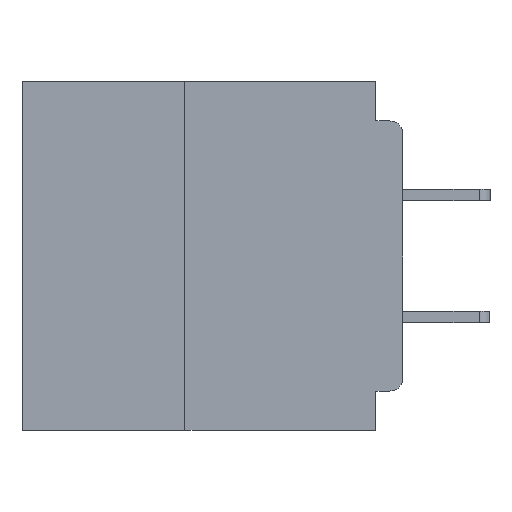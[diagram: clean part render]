
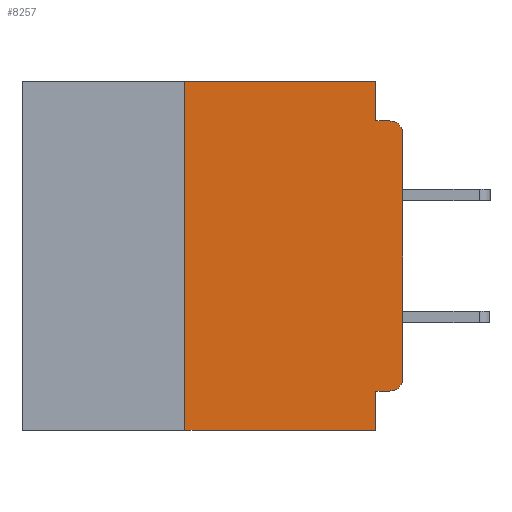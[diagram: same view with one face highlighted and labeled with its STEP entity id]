
A CAD part, left-side view. The second image highlights one B-rep face of the part: STEP entity #8257.
In plain terms, the highlighted planar face has unit normal (-1, 0, 0).
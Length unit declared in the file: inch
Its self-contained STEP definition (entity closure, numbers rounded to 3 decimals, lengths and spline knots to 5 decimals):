
#768 = EDGE_CURVE ( 'NONE', #29755, #1207, #26819, .T. ) ;
#1207 = VERTEX_POINT ( 'NONE', #32233 ) ;
#1720 = VERTEX_POINT ( 'NONE', #8453 ) ;
#1744 = CARTESIAN_POINT ( 'NONE',  ( 0., 0.031, -0.355 ) ) ;
#4543 = EDGE_CURVE ( 'NONE', #17490, #6788, #8308, .T. ) ;
#4868 = CARTESIAN_POINT ( 'NONE',  ( 0., 0., -0.34 ) ) ;
#5256 = ORIENTED_EDGE ( 'NONE', *, *, #768, .F. ) ;
#5502 = CIRCLE ( 'NONE', #35044, 0.015 ) ;
#6087 = LINE ( 'NONE', #44085, #14259 ) ;
#6788 = VERTEX_POINT ( 'NONE', #32227 ) ;
#6913 = ORIENTED_EDGE ( 'NONE', *, *, #19976, .F. ) ;
#7163 = DIRECTION ( 'NONE',  ( 0., 1., 0. ) ) ;
#7928 = VERTEX_POINT ( 'NONE', #41625 ) ;
#8257 = ADVANCED_FACE ( 'NONE', ( #42721 ), #23032, .F. ) ;
#8308 = LINE ( 'NONE', #13569, #34589 ) ;
#8453 = CARTESIAN_POINT ( 'NONE',  ( 0., 0.015, -0.355 ) ) ;
#9027 = VERTEX_POINT ( 'NONE', #23716 ) ;
#9641 = ORIENTED_EDGE ( 'NONE', *, *, #42508, .F. ) ;
#10364 = CARTESIAN_POINT ( 'NONE',  ( 0., 0.031, 0. ) ) ;
#10952 = EDGE_CURVE ( 'NONE', #1720, #43732, #23913, .T. ) ;
#11752 = AXIS2_PLACEMENT_3D ( 'NONE', #19891, #43678, #23328 ) ;
#11834 = EDGE_CURVE ( 'NONE', #1720, #17490, #5502, .T. ) ;
#12180 = VECTOR ( 'NONE', #25509, 39.37008 ) ;
#12613 = DIRECTION ( 'NONE',  ( 0., 0., 1. ) ) ;
#12902 = ORIENTED_EDGE ( 'NONE', *, *, #24576, .T. ) ;
#13569 = CARTESIAN_POINT ( 'NONE',  ( 0., 0., 0. ) ) ;
#14259 = VECTOR ( 'NONE', #30494, 39.37008 ) ;
#16666 = VECTOR ( 'NONE', #38317, 39.37008 ) ;
#17490 = VERTEX_POINT ( 'NONE', #4868 ) ;
#17659 = DIRECTION ( 'NONE',  ( -1., 0., 0. ) ) ;
#17727 = DIRECTION ( 'NONE',  ( 0., 0., 1. ) ) ;
#18200 = CARTESIAN_POINT ( 'NONE',  ( 0., 0.031, -0.045 ) ) ;
#18320 = DIRECTION ( 'NONE',  ( 0., -1., 0. ) ) ;
#18440 = VECTOR ( 'NONE', #18320, 39.37008 ) ;
#19341 = ORIENTED_EDGE ( 'NONE', *, *, #11834, .T. ) ;
#19505 = LINE ( 'NONE', #32071, #18440 ) ;
#19891 = CARTESIAN_POINT ( 'NONE',  ( 0., 0.437, 0. ) ) ;
#19976 = EDGE_CURVE ( 'NONE', #43732, #9027, #6087, .T. ) ;
#20398 = DIRECTION ( 'NONE',  ( -1., 0., 0. ) ) ;
#21410 = EDGE_LOOP ( 'NONE', ( #39601, #22512, #5256, #43775, #9641, #30032, #12902, #6913, #34297, #19341 ) ) ;
#21966 = CIRCLE ( 'NONE', #23890, 0.015 ) ;
#22512 = ORIENTED_EDGE ( 'NONE', *, *, #39303, .T. ) ;
#22692 = CARTESIAN_POINT ( 'NONE',  ( 0., 0.031, 0. ) ) ;
#23032 = PLANE ( 'NONE',  #11752 ) ;
#23328 = DIRECTION ( 'NONE',  ( 0., 0., -1. ) ) ;
#23716 = CARTESIAN_POINT ( 'NONE',  ( 0., 0.031, -0.4 ) ) ;
#23890 = AXIS2_PLACEMENT_3D ( 'NONE', #40852, #20398, #44176 ) ;
#23913 = LINE ( 'NONE', #27755, #24995 ) ;
#24576 = EDGE_CURVE ( 'NONE', #7928, #9027, #39431, .T. ) ;
#24995 = VECTOR ( 'NONE', #7163, 39.37008 ) ;
#25076 = VECTOR ( 'NONE', #17727, 39.37008 ) ;
#25509 = DIRECTION ( 'NONE',  ( 0., -1., 0. ) ) ;
#26819 = LINE ( 'NONE', #38227, #16666 ) ;
#27755 = CARTESIAN_POINT ( 'NONE',  ( 0., 0., -0.355 ) ) ;
#28699 = CARTESIAN_POINT ( 'NONE',  ( 0., 0.25, 0. ) ) ;
#28948 = CARTESIAN_POINT ( 'NONE',  ( 0., 0.437, -0.4 ) ) ;
#29755 = VERTEX_POINT ( 'NONE', #18200 ) ;
#30032 = ORIENTED_EDGE ( 'NONE', *, *, #33732, .F. ) ;
#30494 = DIRECTION ( 'NONE',  ( 0., 0., -1. ) ) ;
#30905 = DIRECTION ( 'NONE',  ( 0., 0., -1. ) ) ;
#31334 = CARTESIAN_POINT ( 'NONE',  ( 0., 0.25, -0.4 ) ) ;
#31995 = LINE ( 'NONE', #10364, #39980 ) ;
#32071 = CARTESIAN_POINT ( 'NONE',  ( 0., 0.437, 0. ) ) ;
#32227 = CARTESIAN_POINT ( 'NONE',  ( 0., 0., -0.06 ) ) ;
#32233 = CARTESIAN_POINT ( 'NONE',  ( 0., 0.015, -0.045 ) ) ;
#33732 = EDGE_CURVE ( 'NONE', #7928, #38427, #35237, .T. ) ;
#34297 = ORIENTED_EDGE ( 'NONE', *, *, #10952, .F. ) ;
#34589 = VECTOR ( 'NONE', #12613, 39.37008 ) ;
#35044 = AXIS2_PLACEMENT_3D ( 'NONE', #38103, #17659, #41507 ) ;
#35237 = LINE ( 'NONE', #31334, #25076 ) ;
#38103 = CARTESIAN_POINT ( 'NONE',  ( 0., 0.015, -0.34 ) ) ;
#38227 = CARTESIAN_POINT ( 'NONE',  ( 0., 0., -0.045 ) ) ;
#38317 = DIRECTION ( 'NONE',  ( 0., -1., 0. ) ) ;
#38427 = VERTEX_POINT ( 'NONE', #28699 ) ;
#38576 = VERTEX_POINT ( 'NONE', #22692 ) ;
#39303 = EDGE_CURVE ( 'NONE', #6788, #1207, #21966, .T. ) ;
#39431 = LINE ( 'NONE', #28948, #12180 ) ;
#39601 = ORIENTED_EDGE ( 'NONE', *, *, #4543, .T. ) ;
#39980 = VECTOR ( 'NONE', #30905, 39.37008 ) ;
#40568 = EDGE_CURVE ( 'NONE', #38576, #29755, #31995, .T. ) ;
#40852 = CARTESIAN_POINT ( 'NONE',  ( 0., 0.015, -0.06 ) ) ;
#41507 = DIRECTION ( 'NONE',  ( 0., 0., -1. ) ) ;
#41625 = CARTESIAN_POINT ( 'NONE',  ( 0., 0.25, -0.4 ) ) ;
#42508 = EDGE_CURVE ( 'NONE', #38427, #38576, #19505, .T. ) ;
#42721 = FACE_OUTER_BOUND ( 'NONE', #21410, .T. ) ;
#43678 = DIRECTION ( 'NONE',  ( 1., 0., 0. ) ) ;
#43732 = VERTEX_POINT ( 'NONE', #1744 ) ;
#43775 = ORIENTED_EDGE ( 'NONE', *, *, #40568, .F. ) ;
#44085 = CARTESIAN_POINT ( 'NONE',  ( 0., 0.031, -0.4 ) ) ;
#44176 = DIRECTION ( 'NONE',  ( 0., 0., -1. ) ) ;
